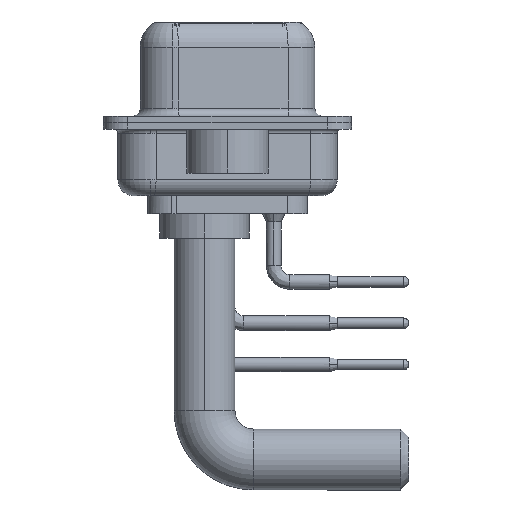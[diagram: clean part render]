
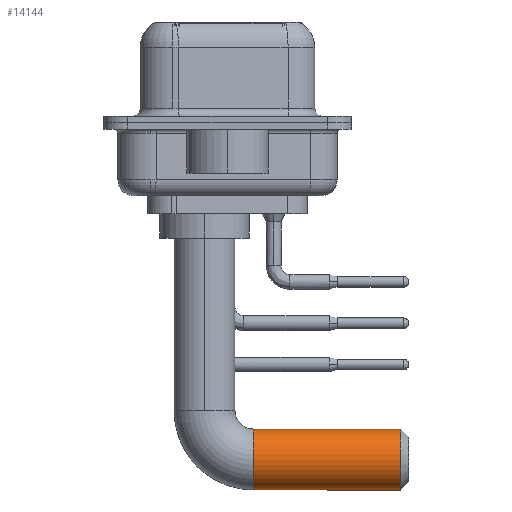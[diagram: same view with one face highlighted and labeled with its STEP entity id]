
A CAD part, left-side view. The second image highlights one B-rep face of the part: STEP entity #14144.
In plain terms, the highlighted cylindrical face has radius 1.875 mm (diameter 3.75 mm), a partial arc.
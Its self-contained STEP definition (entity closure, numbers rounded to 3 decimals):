
#1972 = CARTESIAN_POINT ( 'NONE',  ( 0., -3., -11.755 ) ) ;
#1990 = AXIS2_PLACEMENT_3D ( 'NONE', #19325, #2046, #29351 ) ;
#2046 = DIRECTION ( 'NONE',  ( 0., 1., 0. ) ) ;
#2304 = VERTEX_POINT ( 'NONE', #11119 ) ;
#5726 = LINE ( 'NONE', #30873, #21003 ) ;
#7375 = CARTESIAN_POINT ( 'NONE',  ( 0., -12.07, -11.755 ) ) ;
#7903 = LINE ( 'NONE', #15466, #27764 ) ;
#8849 = VERTEX_POINT ( 'NONE', #1972 ) ;
#9330 = CARTESIAN_POINT ( 'NONE',  ( 0., -3., -13.63 ) ) ;
#10169 = AXIS2_PLACEMENT_3D ( 'NONE', #17427, #18189, #18362 ) ;
#10749 = CARTESIAN_POINT ( 'NONE',  ( 0., -12.07, -15.505 ) ) ;
#11119 = CARTESIAN_POINT ( 'NONE',  ( 0., -3., -15.505 ) ) ;
#11218 = EDGE_CURVE ( 'NONE', #22591, #29568, #16170, .T. ) ;
#14144 = ADVANCED_FACE ( 'NONE', ( #21828 ), #31844, .T. ) ;
#15466 = CARTESIAN_POINT ( 'NONE',  ( 0., -3., -15.505 ) ) ;
#16170 = CIRCLE ( 'NONE', #1990, 1.875 ) ;
#17253 = ORIENTED_EDGE ( 'NONE', *, *, #29470, .T. ) ;
#17427 = CARTESIAN_POINT ( 'NONE',  ( 0., -3., -13.63 ) ) ;
#17955 = DIRECTION ( 'NONE',  ( 0., -1., 0. ) ) ;
#17996 = ORIENTED_EDGE ( 'NONE', *, *, #19850, .T. ) ;
#18189 = DIRECTION ( 'NONE',  ( 0., -1., 0. ) ) ;
#18362 = DIRECTION ( 'NONE',  ( -1., 0., 0. ) ) ;
#19325 = CARTESIAN_POINT ( 'NONE',  ( 0., -12.07, -13.63 ) ) ;
#19377 = DIRECTION ( 'NONE',  ( 0., -1., 0. ) ) ;
#19850 = EDGE_CURVE ( 'NONE', #2304, #22591, #7903, .T. ) ;
#20156 = CIRCLE ( 'NONE', #10169, 1.875 ) ;
#21003 = VECTOR ( 'NONE', #21334, 1000. ) ;
#21334 = DIRECTION ( 'NONE',  ( 0., -1., 0. ) ) ;
#21828 = FACE_OUTER_BOUND ( 'NONE', #31377, .T. ) ;
#22591 = VERTEX_POINT ( 'NONE', #10749 ) ;
#24219 = EDGE_CURVE ( 'NONE', #8849, #29568, #5726, .T. ) ;
#27764 = VECTOR ( 'NONE', #17955, 1000. ) ;
#29351 = DIRECTION ( 'NONE',  ( 0., 0., -1. ) ) ;
#29396 = DIRECTION ( 'NONE',  ( 0., 0., -1. ) ) ;
#29470 = EDGE_CURVE ( 'NONE', #8849, #2304, #20156, .T. ) ;
#29568 = VERTEX_POINT ( 'NONE', #7375 ) ;
#29657 = ORIENTED_EDGE ( 'NONE', *, *, #11218, .T. ) ;
#30873 = CARTESIAN_POINT ( 'NONE',  ( 0., -3., -11.755 ) ) ;
#31377 = EDGE_LOOP ( 'NONE', ( #32188, #17253, #17996, #29657 ) ) ;
#31696 = AXIS2_PLACEMENT_3D ( 'NONE', #9330, #19377, #29396 ) ;
#31844 = CYLINDRICAL_SURFACE ( 'NONE', #31696, 1.875 ) ;
#32188 = ORIENTED_EDGE ( 'NONE', *, *, #24219, .F. ) ;
